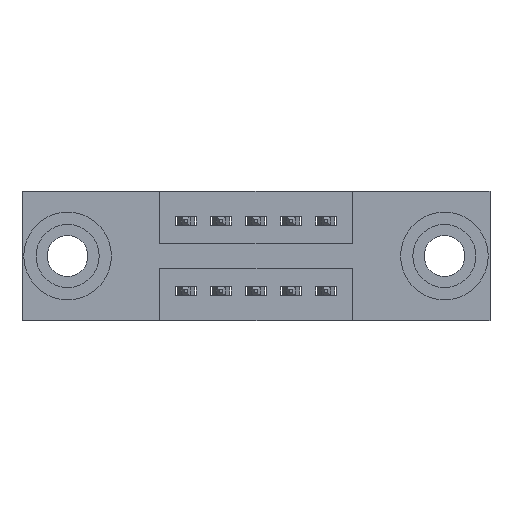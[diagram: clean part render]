
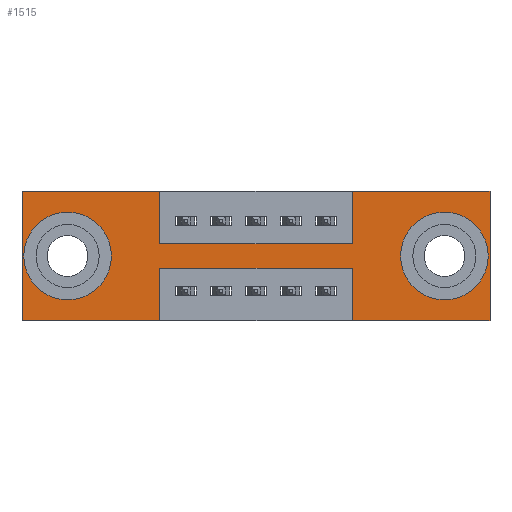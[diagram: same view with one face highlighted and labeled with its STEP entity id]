
A CAD part, front view. The second image highlights one B-rep face of the part: STEP entity #1515.
In plain terms, the highlighted planar face has unit normal (0, -1, 0).
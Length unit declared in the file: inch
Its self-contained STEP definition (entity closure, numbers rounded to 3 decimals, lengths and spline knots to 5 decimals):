
#6 = LINE ( 'NONE', #413, #3936 ) ;
#129 = LINE ( 'NONE', #986, #5791 ) ;
#298 = VERTEX_POINT ( 'NONE', #2994 ) ;
#357 = ORIENTED_EDGE ( 'NONE', *, *, #7753, .F. ) ;
#397 = EDGE_LOOP ( 'NONE', ( #2793, #2833, #5394, #8179, #5200, #357, #4547, #1279, #5874, #1187, #5425, #2113 ) ) ;
#413 = CARTESIAN_POINT ( 'NONE',  ( 0.3925, 0., -0.37 ) ) ;
#510 = CARTESIAN_POINT ( 'NONE',  ( 1.205, 0., -0.185 ) ) ;
#512 = VERTEX_POINT ( 'NONE', #7274 ) ;
#908 = LINE ( 'NONE', #2711, #3409 ) ;
#986 = CARTESIAN_POINT ( 'NONE',  ( 0.3925, 0., 0. ) ) ;
#991 = AXIS2_PLACEMENT_3D ( 'NONE', #3437, #9507, #5650 ) ;
#1028 = CARTESIAN_POINT ( 'NONE',  ( 0.13, 0., -0.263 ) ) ;
#1042 = CARTESIAN_POINT ( 'NONE',  ( 0.3925, 0., -0.22 ) ) ;
#1187 = ORIENTED_EDGE ( 'NONE', *, *, #4091, .F. ) ;
#1279 = ORIENTED_EDGE ( 'NONE', *, *, #2897, .F. ) ;
#1515 = ADVANCED_FACE ( 'NONE', ( #6623, #4211, #4666 ), #3467, .T. ) ;
#1526 = VECTOR ( 'NONE', #6435, 39.37008 ) ;
#1716 = CARTESIAN_POINT ( 'NONE',  ( 0., 0., 0. ) ) ;
#1907 = CARTESIAN_POINT ( 'NONE',  ( 0., 0., -0.37 ) ) ;
#1975 = VERTEX_POINT ( 'NONE', #7464 ) ;
#2113 = ORIENTED_EDGE ( 'NONE', *, *, #5454, .F. ) ;
#2199 = VERTEX_POINT ( 'NONE', #5704 ) ;
#2371 = CARTESIAN_POINT ( 'NONE',  ( 0.13, 0., -0.185 ) ) ;
#2499 = DIRECTION ( 'NONE',  ( -1., 0., 0. ) ) ;
#2500 = EDGE_CURVE ( 'NONE', #6187, #8572, #6251, .T. ) ;
#2621 = CARTESIAN_POINT ( 'NONE',  ( 1.205, 0., -0.185 ) ) ;
#2711 = CARTESIAN_POINT ( 'NONE',  ( 0.9425, 0., 0. ) ) ;
#2793 = ORIENTED_EDGE ( 'NONE', *, *, #3071, .F. ) ;
#2833 = ORIENTED_EDGE ( 'NONE', *, *, #2500, .F. ) ;
#2867 = CARTESIAN_POINT ( 'NONE',  ( 1.205, 0., -0.107 ) ) ;
#2888 = LINE ( 'NONE', #3593, #9369 ) ;
#2897 = EDGE_CURVE ( 'NONE', #2199, #7528, #2888, .T. ) ;
#2938 = CARTESIAN_POINT ( 'NONE',  ( 0.9425, 0., -0.37 ) ) ;
#2994 = CARTESIAN_POINT ( 'NONE',  ( 0.3925, 0., 0. ) ) ;
#2998 = CIRCLE ( 'NONE', #991, 0.078 ) ;
#3071 = EDGE_CURVE ( 'NONE', #8572, #6966, #6, .T. ) ;
#3369 = DIRECTION ( 'NONE',  ( 1., 0., 0. ) ) ;
#3409 = VECTOR ( 'NONE', #7219, 39.37008 ) ;
#3431 = EDGE_CURVE ( 'NONE', #7202, #7555, #4401, .T. ) ;
#3437 = CARTESIAN_POINT ( 'NONE',  ( 0.13, 0., -0.185 ) ) ;
#3467 = PLANE ( 'NONE',  #6304 ) ;
#3512 = AXIS2_PLACEMENT_3D ( 'NONE', #510, #7835, #9279 ) ;
#3593 = CARTESIAN_POINT ( 'NONE',  ( 0.3925, 0., -0.15 ) ) ;
#3600 = CARTESIAN_POINT ( 'NONE',  ( 0.9425, 0., -0.22 ) ) ;
#3609 = CARTESIAN_POINT ( 'NONE',  ( 0.3925, 0., -0.22 ) ) ;
#3936 = VECTOR ( 'NONE', #7035, 39.37008 ) ;
#3941 = LINE ( 'NONE', #1716, #7503 ) ;
#4024 = DIRECTION ( 'NONE',  ( 0., 0., -1. ) ) ;
#4091 = EDGE_CURVE ( 'NONE', #1975, #298, #4961, .T. ) ;
#4211 = FACE_BOUND ( 'NONE', #7757, .T. ) ;
#4244 = CIRCLE ( 'NONE', #6988, 0.078 ) ;
#4274 = CARTESIAN_POINT ( 'NONE',  ( 0., 0., -0.37 ) ) ;
#4279 = ORIENTED_EDGE ( 'NONE', *, *, #7970, .T. ) ;
#4308 = VECTOR ( 'NONE', #2499, 39.37008 ) ;
#4401 = CIRCLE ( 'NONE', #7088, 0.078 ) ;
#4478 = DIRECTION ( 'NONE',  ( 0., 0., 1. ) ) ;
#4547 = ORIENTED_EDGE ( 'NONE', *, *, #9136, .F. ) ;
#4666 = FACE_OUTER_BOUND ( 'NONE', #397, .T. ) ;
#4825 = EDGE_CURVE ( 'NONE', #9247, #1975, #7351, .T. ) ;
#4910 = EDGE_LOOP ( 'NONE', ( #6510, #6607 ) ) ;
#4912 = VERTEX_POINT ( 'NONE', #8200 ) ;
#4936 = VECTOR ( 'NONE', #9490, 39.37008 ) ;
#4961 = LINE ( 'NONE', #7762, #7702 ) ;
#5085 = CARTESIAN_POINT ( 'NONE',  ( 0.9425, 0., -0.15 ) ) ;
#5189 = EDGE_CURVE ( 'NONE', #7181, #7962, #4244, .T. ) ;
#5200 = ORIENTED_EDGE ( 'NONE', *, *, #8235, .F. ) ;
#5218 = CARTESIAN_POINT ( 'NONE',  ( 0., 0., 0. ) ) ;
#5379 = CARTESIAN_POINT ( 'NONE',  ( 0.9425, 0., 0. ) ) ;
#5394 = ORIENTED_EDGE ( 'NONE', *, *, #7265, .F. ) ;
#5409 = VECTOR ( 'NONE', #4478, 39.37008 ) ;
#5425 = ORIENTED_EDGE ( 'NONE', *, *, #4825, .F. ) ;
#5454 = EDGE_CURVE ( 'NONE', #6966, #9247, #6764, .T. ) ;
#5614 = DIRECTION ( 'NONE',  ( 0., 0., -1. ) ) ;
#5650 = DIRECTION ( 'NONE',  ( 0., 0., 1. ) ) ;
#5704 = CARTESIAN_POINT ( 'NONE',  ( 0.3925, 0., -0.15 ) ) ;
#5791 = VECTOR ( 'NONE', #4024, 39.37008 ) ;
#5798 = CARTESIAN_POINT ( 'NONE',  ( 0., 0., -0.37 ) ) ;
#5874 = ORIENTED_EDGE ( 'NONE', *, *, #7694, .F. ) ;
#6187 = VERTEX_POINT ( 'NONE', #3600 ) ;
#6251 = LINE ( 'NONE', #1042, #4308 ) ;
#6304 = AXIS2_PLACEMENT_3D ( 'NONE', #4274, #8737, #9461 ) ;
#6392 = CARTESIAN_POINT ( 'NONE',  ( 0.13, 0., -0.107 ) ) ;
#6435 = DIRECTION ( 'NONE',  ( 0., 0., -1. ) ) ;
#6510 = ORIENTED_EDGE ( 'NONE', *, *, #8220, .T. ) ;
#6563 = DIRECTION ( 'NONE',  ( 0., 0., 1. ) ) ;
#6607 = ORIENTED_EDGE ( 'NONE', *, *, #3431, .T. ) ;
#6623 = FACE_BOUND ( 'NONE', #4910, .T. ) ;
#6764 = LINE ( 'NONE', #5798, #4936 ) ;
#6799 = LINE ( 'NONE', #7090, #1526 ) ;
#6817 = DIRECTION ( 'NONE',  ( 1., 0., 0. ) ) ;
#6840 = CARTESIAN_POINT ( 'NONE',  ( 1.335, 0., -0.37 ) ) ;
#6858 = DIRECTION ( 'NONE',  ( 0., 0., 1. ) ) ;
#6966 = VERTEX_POINT ( 'NONE', #8365 ) ;
#6988 = AXIS2_PLACEMENT_3D ( 'NONE', #2371, #8372, #6858 ) ;
#7035 = DIRECTION ( 'NONE',  ( 0., 0., -1. ) ) ;
#7046 = LINE ( 'NONE', #2938, #7147 ) ;
#7088 = AXIS2_PLACEMENT_3D ( 'NONE', #2621, #8543, #5614 ) ;
#7090 = CARTESIAN_POINT ( 'NONE',  ( 1.335, 0., 0. ) ) ;
#7147 = VECTOR ( 'NONE', #6563, 39.37008 ) ;
#7181 = VERTEX_POINT ( 'NONE', #1028 ) ;
#7202 = VERTEX_POINT ( 'NONE', #9317 ) ;
#7219 = DIRECTION ( 'NONE',  ( 0., 0., 1. ) ) ;
#7265 = EDGE_CURVE ( 'NONE', #512, #6187, #7046, .T. ) ;
#7274 = CARTESIAN_POINT ( 'NONE',  ( 0.9425, 0., -0.37 ) ) ;
#7351 = LINE ( 'NONE', #5218, #5409 ) ;
#7464 = CARTESIAN_POINT ( 'NONE',  ( 0., 0., 0. ) ) ;
#7503 = VECTOR ( 'NONE', #7579, 39.37008 ) ;
#7528 = VERTEX_POINT ( 'NONE', #5085 ) ;
#7555 = VERTEX_POINT ( 'NONE', #2867 ) ;
#7574 = ORIENTED_EDGE ( 'NONE', *, *, #5189, .T. ) ;
#7579 = DIRECTION ( 'NONE',  ( 1., 0., 0. ) ) ;
#7694 = EDGE_CURVE ( 'NONE', #298, #2199, #129, .T. ) ;
#7702 = VECTOR ( 'NONE', #3369, 39.37008 ) ;
#7753 = EDGE_CURVE ( 'NONE', #7811, #4912, #3941, .T. ) ;
#7757 = EDGE_LOOP ( 'NONE', ( #4279, #7574 ) ) ;
#7762 = CARTESIAN_POINT ( 'NONE',  ( 0., 0., 0. ) ) ;
#7811 = VERTEX_POINT ( 'NONE', #5379 ) ;
#7835 = DIRECTION ( 'NONE',  ( 0., 1., 0. ) ) ;
#7879 = EDGE_CURVE ( 'NONE', #8494, #512, #8657, .T. ) ;
#7962 = VERTEX_POINT ( 'NONE', #6392 ) ;
#7970 = EDGE_CURVE ( 'NONE', #7962, #7181, #2998, .T. ) ;
#8066 = CARTESIAN_POINT ( 'NONE',  ( 0., 0., -0.37 ) ) ;
#8179 = ORIENTED_EDGE ( 'NONE', *, *, #7879, .F. ) ;
#8200 = CARTESIAN_POINT ( 'NONE',  ( 1.335, 0., 0. ) ) ;
#8220 = EDGE_CURVE ( 'NONE', #7555, #7202, #8883, .T. ) ;
#8235 = EDGE_CURVE ( 'NONE', #4912, #8494, #6799, .T. ) ;
#8365 = CARTESIAN_POINT ( 'NONE',  ( 0.3925, 0., -0.37 ) ) ;
#8372 = DIRECTION ( 'NONE',  ( 0., 1., 0. ) ) ;
#8494 = VERTEX_POINT ( 'NONE', #6840 ) ;
#8543 = DIRECTION ( 'NONE',  ( 0., 1., 0. ) ) ;
#8572 = VERTEX_POINT ( 'NONE', #3609 ) ;
#8657 = LINE ( 'NONE', #1907, #8774 ) ;
#8737 = DIRECTION ( 'NONE',  ( 0., -1., 0. ) ) ;
#8774 = VECTOR ( 'NONE', #9204, 39.37008 ) ;
#8883 = CIRCLE ( 'NONE', #3512, 0.078 ) ;
#9136 = EDGE_CURVE ( 'NONE', #7528, #7811, #908, .T. ) ;
#9204 = DIRECTION ( 'NONE',  ( -1., 0., 0. ) ) ;
#9247 = VERTEX_POINT ( 'NONE', #8066 ) ;
#9279 = DIRECTION ( 'NONE',  ( 0., 0., -1. ) ) ;
#9317 = CARTESIAN_POINT ( 'NONE',  ( 1.205, 0., -0.263 ) ) ;
#9369 = VECTOR ( 'NONE', #6817, 39.37008 ) ;
#9461 = DIRECTION ( 'NONE',  ( 0., 0., -1. ) ) ;
#9490 = DIRECTION ( 'NONE',  ( -1., 0., 0. ) ) ;
#9507 = DIRECTION ( 'NONE',  ( 0., 1., 0. ) ) ;
